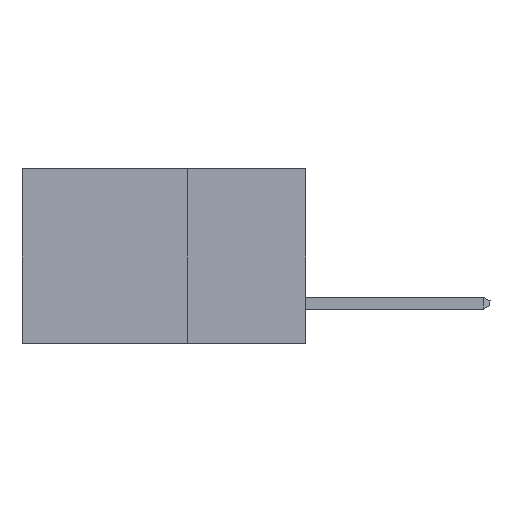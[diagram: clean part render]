
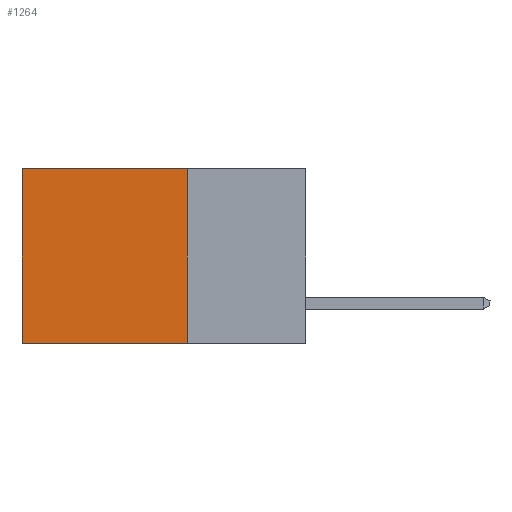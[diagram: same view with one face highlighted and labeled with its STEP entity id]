
A CAD part, left-side view. The second image highlights one B-rep face of the part: STEP entity #1264.
In plain terms, the highlighted planar face has unit normal (-1, 0, 0).
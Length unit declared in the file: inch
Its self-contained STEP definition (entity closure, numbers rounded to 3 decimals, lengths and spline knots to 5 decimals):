
#68 = EDGE_CURVE ( 'NONE', #7868, #4253, #5671, .T. ) ;
#86 = CARTESIAN_POINT ( 'NONE',  ( 0.2615, 0.25, -0.37 ) ) ;
#1120 = VERTEX_POINT ( 'NONE', #9442 ) ;
#1181 = VERTEX_POINT ( 'NONE', #2754 ) ;
#1264 = ADVANCED_FACE ( 'NONE', ( #8020 ), #3676, .F. ) ;
#1296 = VECTOR ( 'NONE', #2775, 39.37008 ) ;
#1415 = CARTESIAN_POINT ( 'NONE',  ( 0.2615, 0.25, -0.37 ) ) ;
#1588 = ORIENTED_EDGE ( 'NONE', *, *, #4161, .T. ) ;
#1722 = LINE ( 'NONE', #5311, #7350 ) ;
#2297 = EDGE_CURVE ( 'NONE', #1120, #4253, #1722, .T. ) ;
#2747 = CARTESIAN_POINT ( 'NONE',  ( 0.2615, 0.6, 0. ) ) ;
#2754 = CARTESIAN_POINT ( 'NONE',  ( 0.2615, 0.25, 0. ) ) ;
#2755 = ORIENTED_EDGE ( 'NONE', *, *, #6212, .F. ) ;
#2775 = DIRECTION ( 'NONE',  ( 0., 1., 0. ) ) ;
#3620 = DIRECTION ( 'NONE',  ( 1., 0., 0. ) ) ;
#3676 = PLANE ( 'NONE',  #6603 ) ;
#4026 = LINE ( 'NONE', #5434, #1296 ) ;
#4161 = EDGE_CURVE ( 'NONE', #1181, #7868, #4026, .T. ) ;
#4253 = VERTEX_POINT ( 'NONE', #4304 ) ;
#4304 = CARTESIAN_POINT ( 'NONE',  ( 0.2615, 0.6, -0.37 ) ) ;
#4387 = DIRECTION ( 'NONE',  ( 0., 1., 0. ) ) ;
#4631 = EDGE_LOOP ( 'NONE', ( #9788, #10118, #2755, #1588 ) ) ;
#4688 = DIRECTION ( 'NONE',  ( 0., 0., -1. ) ) ;
#5311 = CARTESIAN_POINT ( 'NONE',  ( 0.2615, 0.25, -0.37 ) ) ;
#5434 = CARTESIAN_POINT ( 'NONE',  ( 0.2615, 0.25, 0. ) ) ;
#5671 = LINE ( 'NONE', #9122, #11421 ) ;
#6212 = EDGE_CURVE ( 'NONE', #1181, #1120, #11001, .T. ) ;
#6293 = DIRECTION ( 'NONE',  ( 0., 0., -1. ) ) ;
#6603 = AXIS2_PLACEMENT_3D ( 'NONE', #86, #3620, #6293 ) ;
#7350 = VECTOR ( 'NONE', #4387, 39.37008 ) ;
#7493 = DIRECTION ( 'NONE',  ( 0., 0., -1. ) ) ;
#7868 = VERTEX_POINT ( 'NONE', #2747 ) ;
#8020 = FACE_OUTER_BOUND ( 'NONE', #4631, .T. ) ;
#9122 = CARTESIAN_POINT ( 'NONE',  ( 0.2615, 0.6, -0.37 ) ) ;
#9442 = CARTESIAN_POINT ( 'NONE',  ( 0.2615, 0.25, -0.37 ) ) ;
#9788 = ORIENTED_EDGE ( 'NONE', *, *, #68, .T. ) ;
#10040 = VECTOR ( 'NONE', #7493, 39.37008 ) ;
#10118 = ORIENTED_EDGE ( 'NONE', *, *, #2297, .F. ) ;
#11001 = LINE ( 'NONE', #1415, #10040 ) ;
#11421 = VECTOR ( 'NONE', #4688, 39.37008 ) ;
